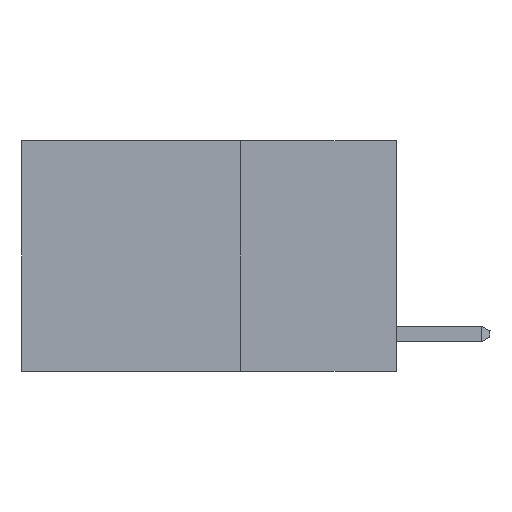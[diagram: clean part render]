
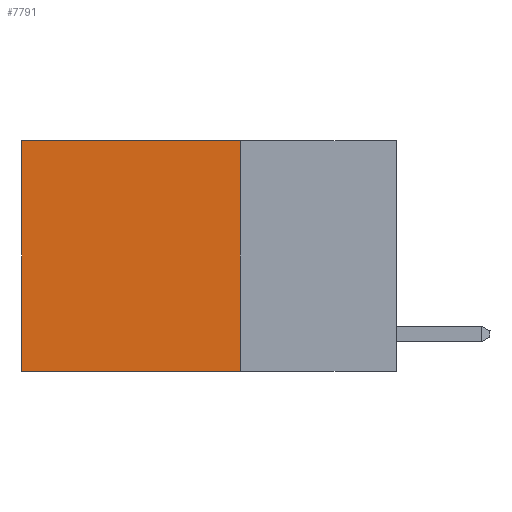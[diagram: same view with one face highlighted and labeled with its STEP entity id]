
A CAD part, left-side view. The second image highlights one B-rep face of the part: STEP entity #7791.
In plain terms, the highlighted planar face has unit normal (-1, 0, 0).
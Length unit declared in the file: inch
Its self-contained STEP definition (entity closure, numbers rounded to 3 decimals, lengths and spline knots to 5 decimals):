
#127 = EDGE_CURVE ( 'NONE', #685, #12816, #11867, .T. ) ;
#552 = CARTESIAN_POINT ( 'NONE',  ( 0.2625, 0.25, 0. ) ) ;
#685 = VERTEX_POINT ( 'NONE', #15772 ) ;
#986 = VECTOR ( 'NONE', #8246, 39.37008 ) ;
#1430 = PLANE ( 'NONE',  #8063 ) ;
#1686 = EDGE_CURVE ( 'NONE', #9636, #3273, #2829, .T. ) ;
#1958 = ORIENTED_EDGE ( 'NONE', *, *, #1686, .T. ) ;
#2829 = LINE ( 'NONE', #5689, #986 ) ;
#3091 = VECTOR ( 'NONE', #5705, 39.37008 ) ;
#3273 = VERTEX_POINT ( 'NONE', #8200 ) ;
#3650 = EDGE_CURVE ( 'NONE', #685, #9636, #15914, .T. ) ;
#3824 = DIRECTION ( 'NONE',  ( 0., 0., -1. ) ) ;
#3978 = CARTESIAN_POINT ( 'NONE',  ( 0.2625, 0.25, -0.37 ) ) ;
#4593 = ORIENTED_EDGE ( 'NONE', *, *, #3650, .T. ) ;
#5177 = DIRECTION ( 'NONE',  ( 0., 0., -1. ) ) ;
#5340 = CARTESIAN_POINT ( 'NONE',  ( 0.2625, 0.25, 0. ) ) ;
#5689 = CARTESIAN_POINT ( 'NONE',  ( 0.2625, 0.6, 0. ) ) ;
#5705 = DIRECTION ( 'NONE',  ( 0., 1., 0. ) ) ;
#5786 = LINE ( 'NONE', #11996, #14900 ) ;
#7594 = ORIENTED_EDGE ( 'NONE', *, *, #10053, .F. ) ;
#7791 = ADVANCED_FACE ( 'NONE', ( #14179 ), #1430, .F. ) ;
#8063 = AXIS2_PLACEMENT_3D ( 'NONE', #5340, #16748, #3824 ) ;
#8200 = CARTESIAN_POINT ( 'NONE',  ( 0.2625, 0.6, -0.37 ) ) ;
#8246 = DIRECTION ( 'NONE',  ( 0., 0., -1. ) ) ;
#8633 = ORIENTED_EDGE ( 'NONE', *, *, #127, .F. ) ;
#9636 = VERTEX_POINT ( 'NONE', #14911 ) ;
#10053 = EDGE_CURVE ( 'NONE', #12816, #3273, #5786, .T. ) ;
#11231 = EDGE_LOOP ( 'NONE', ( #1958, #7594, #8633, #4593 ) ) ;
#11867 = LINE ( 'NONE', #14266, #16764 ) ;
#11996 = CARTESIAN_POINT ( 'NONE',  ( 0.2625, 0.25, -0.37 ) ) ;
#12816 = VERTEX_POINT ( 'NONE', #3978 ) ;
#14179 = FACE_OUTER_BOUND ( 'NONE', #11231, .T. ) ;
#14266 = CARTESIAN_POINT ( 'NONE',  ( 0.2625, 0.25, 0. ) ) ;
#14474 = DIRECTION ( 'NONE',  ( 0., 1., 0. ) ) ;
#14900 = VECTOR ( 'NONE', #14474, 39.37008 ) ;
#14911 = CARTESIAN_POINT ( 'NONE',  ( 0.2625, 0.6, 0. ) ) ;
#15772 = CARTESIAN_POINT ( 'NONE',  ( 0.2625, 0.25, 0. ) ) ;
#15914 = LINE ( 'NONE', #552, #3091 ) ;
#16748 = DIRECTION ( 'NONE',  ( 1., 0., 0. ) ) ;
#16764 = VECTOR ( 'NONE', #5177, 39.37008 ) ;
